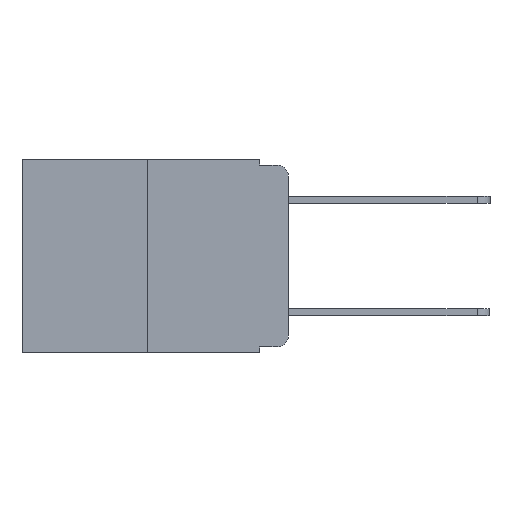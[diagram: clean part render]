
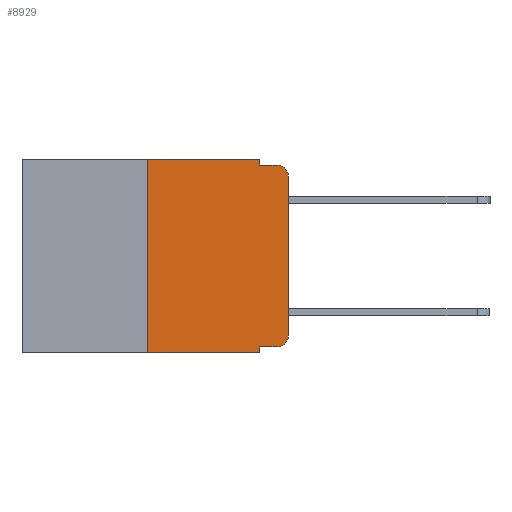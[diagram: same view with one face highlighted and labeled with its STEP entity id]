
A CAD part, left-side view. The second image highlights one B-rep face of the part: STEP entity #8929.
In plain terms, the highlighted planar face has unit normal (-1, 0, 0).
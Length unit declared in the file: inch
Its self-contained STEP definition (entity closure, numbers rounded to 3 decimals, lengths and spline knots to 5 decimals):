
#64 = AXIS2_PLACEMENT_3D ( 'NONE', #11060, #5256, #11981 ) ;
#175 = LINE ( 'NONE', #4897, #6257 ) ;
#347 = CARTESIAN_POINT ( 'NONE',  ( 0., 0.051, -0.343 ) ) ;
#492 = EDGE_CURVE ( 'NONE', #6021, #5189, #10418, .T. ) ;
#726 = EDGE_CURVE ( 'NONE', #6308, #6021, #7179, .T. ) ;
#761 = ORIENTED_EDGE ( 'NONE', *, *, #3527, .T. ) ;
#1185 = ORIENTED_EDGE ( 'NONE', *, *, #492, .F. ) ;
#1190 = DIRECTION ( 'NONE',  ( 0., 0., 1. ) ) ;
#1565 = ORIENTED_EDGE ( 'NONE', *, *, #4667, .F. ) ;
#1718 = CARTESIAN_POINT ( 'NONE',  ( 0., 0.051, 0. ) ) ;
#2310 = VERTEX_POINT ( 'NONE', #5510 ) ;
#2339 = ORIENTED_EDGE ( 'NONE', *, *, #2972, .F. ) ;
#2402 = DIRECTION ( 'NONE',  ( 0., -1., 0. ) ) ;
#2888 = VERTEX_POINT ( 'NONE', #11269 ) ;
#2972 = EDGE_CURVE ( 'NONE', #6154, #5148, #3607, .T. ) ;
#3095 = EDGE_CURVE ( 'NONE', #6491, #5148, #11469, .T. ) ;
#3170 = LINE ( 'NONE', #12070, #9168 ) ;
#3177 = DIRECTION ( 'NONE',  ( 0., 0., 1. ) ) ;
#3527 = EDGE_CURVE ( 'NONE', #7167, #3601, #11723, .T. ) ;
#3601 = VERTEX_POINT ( 'NONE', #5309 ) ;
#3607 = LINE ( 'NONE', #11524, #11322 ) ;
#3926 = CARTESIAN_POINT ( 'NONE',  ( 0., 0.473, -0.343 ) ) ;
#4203 = CARTESIAN_POINT ( 'NONE',  ( 0., 0.02, -0.01 ) ) ;
#4303 = DIRECTION ( 'NONE',  ( -1., 0., 0. ) ) ;
#4320 = DIRECTION ( 'NONE',  ( 0., -1., 0. ) ) ;
#4349 = AXIS2_PLACEMENT_3D ( 'NONE', #10305, #4303, #11223 ) ;
#4402 = CARTESIAN_POINT ( 'NONE',  ( 0., 0.25, 0. ) ) ;
#4505 = EDGE_CURVE ( 'NONE', #6491, #2888, #7713, .T. ) ;
#4667 = EDGE_CURVE ( 'NONE', #2888, #6308, #175, .T. ) ;
#4727 = DIRECTION ( 'NONE',  ( 0., 0., -1. ) ) ;
#4756 = CARTESIAN_POINT ( 'NONE',  ( 0., 0.25, -0.343 ) ) ;
#4897 = CARTESIAN_POINT ( 'NONE',  ( 0., 0.473, 0. ) ) ;
#5148 = VERTEX_POINT ( 'NONE', #347 ) ;
#5162 = EDGE_CURVE ( 'NONE', #6154, #2310, #3170, .T. ) ;
#5189 = VERTEX_POINT ( 'NONE', #4203 ) ;
#5256 = DIRECTION ( 'NONE',  ( 1., 0., 0. ) ) ;
#5309 = CARTESIAN_POINT ( 'NONE',  ( 0., 0., -0.03 ) ) ;
#5510 = CARTESIAN_POINT ( 'NONE',  ( 0., 0.02, -0.333 ) ) ;
#5536 = ORIENTED_EDGE ( 'NONE', *, *, #5162, .T. ) ;
#6021 = VERTEX_POINT ( 'NONE', #11086 ) ;
#6121 = CIRCLE ( 'NONE', #4349, 0.02 ) ;
#6154 = VERTEX_POINT ( 'NONE', #7563 ) ;
#6190 = EDGE_LOOP ( 'NONE', ( #761, #7039, #1185, #7345, #1565, #12542, #12819, #2339, #5536, #10691 ) ) ;
#6257 = VECTOR ( 'NONE', #2402, 39.37008 ) ;
#6308 = VERTEX_POINT ( 'NONE', #13211 ) ;
#6384 = EDGE_CURVE ( 'NONE', #3601, #5189, #12965, .T. ) ;
#6408 = DIRECTION ( 'NONE',  ( 0., -1., 0. ) ) ;
#6491 = VERTEX_POINT ( 'NONE', #4756 ) ;
#6827 = CARTESIAN_POINT ( 'NONE',  ( 0., 0.02, -0.03 ) ) ;
#6868 = VECTOR ( 'NONE', #10113, 39.37008 ) ;
#7039 = ORIENTED_EDGE ( 'NONE', *, *, #6384, .T. ) ;
#7167 = VERTEX_POINT ( 'NONE', #11150 ) ;
#7179 = LINE ( 'NONE', #1718, #6868 ) ;
#7239 = DIRECTION ( 'NONE',  ( 0., -1., 0. ) ) ;
#7345 = ORIENTED_EDGE ( 'NONE', *, *, #726, .F. ) ;
#7563 = CARTESIAN_POINT ( 'NONE',  ( 0., 0.051, -0.333 ) ) ;
#7713 = LINE ( 'NONE', #4402, #9049 ) ;
#7808 = DIRECTION ( 'NONE',  ( 0., 0., -1. ) ) ;
#8019 = CARTESIAN_POINT ( 'NONE',  ( 0., 0., 0. ) ) ;
#8929 = ADVANCED_FACE ( 'NONE', ( #12618 ), #9240, .F. ) ;
#9049 = VECTOR ( 'NONE', #3177, 39.37008 ) ;
#9062 = EDGE_CURVE ( 'NONE', #2310, #7167, #6121, .T. ) ;
#9168 = VECTOR ( 'NONE', #6408, 39.37008 ) ;
#9240 = PLANE ( 'NONE',  #64 ) ;
#9576 = VECTOR ( 'NONE', #1190, 39.37008 ) ;
#10113 = DIRECTION ( 'NONE',  ( 0., 0., -1. ) ) ;
#10305 = CARTESIAN_POINT ( 'NONE',  ( 0., 0.02, -0.313 ) ) ;
#10418 = LINE ( 'NONE', #13208, #12547 ) ;
#10691 = ORIENTED_EDGE ( 'NONE', *, *, #9062, .T. ) ;
#11060 = CARTESIAN_POINT ( 'NONE',  ( 0., 0.473, 0. ) ) ;
#11086 = CARTESIAN_POINT ( 'NONE',  ( 0., 0.051, -0.01 ) ) ;
#11150 = CARTESIAN_POINT ( 'NONE',  ( 0., 0., -0.313 ) ) ;
#11160 = VECTOR ( 'NONE', #7239, 39.37008 ) ;
#11223 = DIRECTION ( 'NONE',  ( 0., 0., -1. ) ) ;
#11269 = CARTESIAN_POINT ( 'NONE',  ( 0., 0.25, 0. ) ) ;
#11283 = AXIS2_PLACEMENT_3D ( 'NONE', #6827, #13298, #7808 ) ;
#11322 = VECTOR ( 'NONE', #4727, 39.37008 ) ;
#11469 = LINE ( 'NONE', #3926, #11160 ) ;
#11524 = CARTESIAN_POINT ( 'NONE',  ( 0., 0.051, 0. ) ) ;
#11723 = LINE ( 'NONE', #8019, #9576 ) ;
#11981 = DIRECTION ( 'NONE',  ( 0., 0., -1. ) ) ;
#12070 = CARTESIAN_POINT ( 'NONE',  ( 0., 0.051, -0.333 ) ) ;
#12542 = ORIENTED_EDGE ( 'NONE', *, *, #4505, .F. ) ;
#12547 = VECTOR ( 'NONE', #4320, 39.37008 ) ;
#12618 = FACE_OUTER_BOUND ( 'NONE', #6190, .T. ) ;
#12819 = ORIENTED_EDGE ( 'NONE', *, *, #3095, .T. ) ;
#12965 = CIRCLE ( 'NONE', #11283, 0.02 ) ;
#13208 = CARTESIAN_POINT ( 'NONE',  ( 0., 0.051, -0.01 ) ) ;
#13211 = CARTESIAN_POINT ( 'NONE',  ( 0., 0.051, 0. ) ) ;
#13298 = DIRECTION ( 'NONE',  ( -1., 0., 0. ) ) ;
